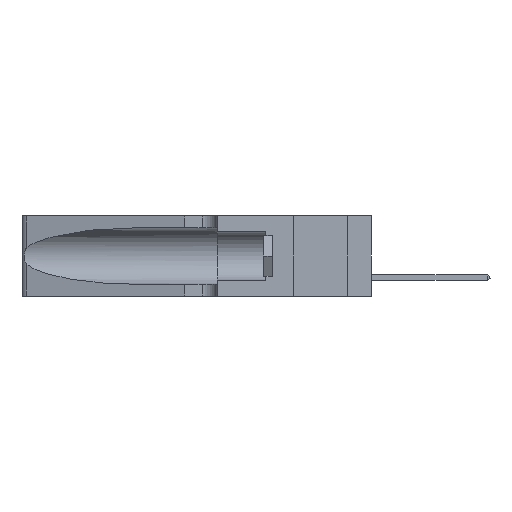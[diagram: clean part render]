
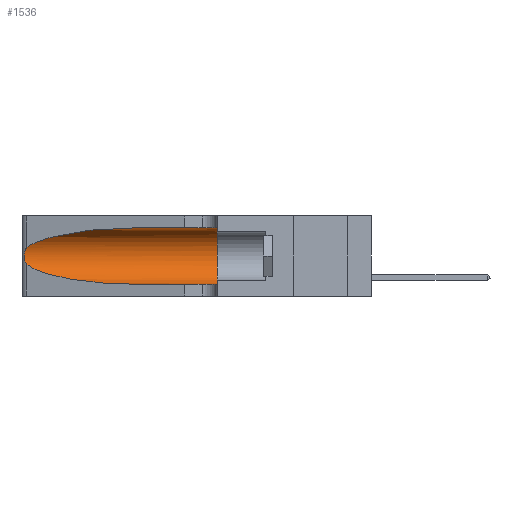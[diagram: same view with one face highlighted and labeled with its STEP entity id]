
A CAD part, left-side view. The second image highlights one B-rep face of the part: STEP entity #1536.
In plain terms, the highlighted cylindrical face has radius 3.308 mm (diameter 6.617 mm), a partial arc.
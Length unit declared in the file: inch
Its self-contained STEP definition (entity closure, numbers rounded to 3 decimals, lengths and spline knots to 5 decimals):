
#342 = CIRCLE ( 'NONE', #3537, 0.13025 ) ;
#1350 = EDGE_CURVE ( 'NONE', #8783, #22635, #342, .T. ) ;
#1366 = CARTESIAN_POINT ( 'NONE',  ( 0.1305, 0.35, 0.05475 ) ) ;
#1536 = ADVANCED_FACE ( 'NONE', ( #18230 ), #26900, .F. ) ;
#2215 = VERTEX_POINT ( 'NONE', #22317 ) ;
#2694 = CARTESIAN_POINT ( 'NONE',  ( 0.2373, 1.15595, 0.28018 ) ) ;
#3537 = AXIS2_PLACEMENT_3D ( 'NONE', #14195, #28420, #31105 ) ;
#4335 = EDGE_CURVE ( 'NONE', #12431, #22635, #7049, .T. ) ;
#4605 = CARTESIAN_POINT ( 'NONE',  ( 0.25487, 1.22718, 0.22369 ) ) ;
#4709 = VERTEX_POINT ( 'NONE', #4605 ) ;
#5006 = LINE ( 'NONE', #28798, #22879 ) ;
#6107 = EDGE_CURVE ( 'NONE', #7689, #8783, #5006, .T. ) ;
#6124 = CARTESIAN_POINT ( 'NONE',  ( 0.25789, 1.23486, 0.15765 ) ) ;
#6458 = CARTESIAN_POINT ( 'NONE',  ( 0.25854, 1.2359, 0.20912 ) ) ;
#6607 = EDGE_CURVE ( 'NONE', #7689, #4709, #11558, .T. ) ;
#7049 = LINE ( 'NONE', #31256, #7746 ) ;
#7689 = VERTEX_POINT ( 'NONE', #12386 ) ;
#7746 = VECTOR ( 'NONE', #16591, 39.37008 ) ;
#7882 = CARTESIAN_POINT ( 'NONE',  ( 0.18966, 0.96281, 0.05475 ) ) ;
#8782 = CARTESIAN_POINT ( 'NONE',  ( 0.25787, 1.23484, 0.2124 ) ) ;
#8783 = VERTEX_POINT ( 'NONE', #11712 ) ;
#10877 = CARTESIAN_POINT ( 'NONE',  ( 0.25555, 1.22993, 0.14849 ) ) ;
#11089 = CARTESIAN_POINT ( 'NONE',  ( 0.25639, 1.23184, 0.21858 ) ) ;
#11193 = CARTESIAN_POINT ( 'NONE',  ( 0.25639, 1.23186, 0.15144 ) ) ;
#11558 =( BOUNDED_CURVE ( )  B_SPLINE_CURVE ( 3, ( #31203, #24676, #2694, #17428 ),
 .UNSPECIFIED., .F., .F. ) 
 B_SPLINE_CURVE_WITH_KNOTS ( ( 4, 4 ),
 ( 1.5708, 2.84003 ),
 .UNSPECIFIED. ) 
 CURVE ( )  GEOMETRIC_REPRESENTATION_ITEM ( )  RATIONAL_B_SPLINE_CURVE ( ( 1., 0.87, 0.87, 1. ) ) 
 REPRESENTATION_ITEM ( '' )  );
#11678 = ORIENTED_EDGE ( 'NONE', *, *, #29140, .T. ) ;
#11712 = CARTESIAN_POINT ( 'NONE',  ( 0.1305, 0.35, 0.31525 ) ) ;
#11810 = ORIENTED_EDGE ( 'NONE', *, *, #21316, .T. ) ;
#12386 = CARTESIAN_POINT ( 'NONE',  ( 0.1305, 0.72297, 0.31525 ) ) ;
#12431 = VERTEX_POINT ( 'NONE', #30463 ) ;
#13354 = ORIENTED_EDGE ( 'NONE', *, *, #1350, .F. ) ;
#13398 = CARTESIAN_POINT ( 'NONE',  ( 0.25487, 1.22718, 0.14631 ) ) ;
#14097 = CARTESIAN_POINT ( 'NONE',  ( 0.1305, 1.61858, 0.185 ) ) ;
#14195 = CARTESIAN_POINT ( 'NONE',  ( 0.1305, 0.35, 0.185 ) ) ;
#14213 = DIRECTION ( 'NONE',  ( 0., -1., 0. ) ) ;
#14747 = CARTESIAN_POINT ( 'NONE',  ( 0.2373, 1.15595, 0.08982 ) ) ;
#15059 = AXIS2_PLACEMENT_3D ( 'NONE', #14097, #14213, #19146 ) ;
#16081 = CARTESIAN_POINT ( 'NONE',  ( 0.25856, 1.23593, 0.16098 ) ) ;
#16591 = DIRECTION ( 'NONE',  ( 0., -1., 0. ) ) ;
#16883 = DIRECTION ( 'NONE',  ( 0., -1., 0. ) ) ;
#17168 = B_SPLINE_CURVE_WITH_KNOTS ( 'NONE', 3,
 ( #23561, #28182, #11089, #8782, #6458, #23456, #30642, #20655, #25415, #16081, #6124, #11193, #10877, #13398 ),
 .UNSPECIFIED., .F., .F.,
 ( 4, 2, 2, 2, 2, 2, 4 ),
 ( 0., 0.00027, 0.00053, 0.00107, 0.0016, 0.00187, 0.00214 ),
 .UNSPECIFIED. ) ;
#17428 = CARTESIAN_POINT ( 'NONE',  ( 0.25487, 1.22718, 0.22369 ) ) ;
#18230 = FACE_OUTER_BOUND ( 'NONE', #22484, .T. ) ;
#19146 = DIRECTION ( 'NONE',  ( 0., 0., -1. ) ) ;
#20655 = CARTESIAN_POINT ( 'NONE',  ( 0.26075, 1.23896, 0.178 ) ) ;
#21316 = EDGE_CURVE ( 'NONE', #2215, #12431, #23280, .T. ) ;
#22025 = CARTESIAN_POINT ( 'NONE',  ( 0.25487, 1.22718, 0.14631 ) ) ;
#22317 = CARTESIAN_POINT ( 'NONE',  ( 0.25487, 1.22718, 0.14631 ) ) ;
#22484 = EDGE_LOOP ( 'NONE', ( #31211, #11678, #11810, #25449, #13354, #24732 ) ) ;
#22635 = VERTEX_POINT ( 'NONE', #1366 ) ;
#22879 = VECTOR ( 'NONE', #16883, 39.37008 ) ;
#23280 =( BOUNDED_CURVE ( )  B_SPLINE_CURVE ( 3, ( #22025, #14747, #7882, #24868 ),
 .UNSPECIFIED., .F., .F. ) 
 B_SPLINE_CURVE_WITH_KNOTS ( ( 4, 4 ),
 ( 3.44316, 4.71239 ),
 .UNSPECIFIED. ) 
 CURVE ( )  GEOMETRIC_REPRESENTATION_ITEM ( )  RATIONAL_B_SPLINE_CURVE ( ( 1., 0.87, 0.87, 1. ) ) 
 REPRESENTATION_ITEM ( '' )  );
#23456 = CARTESIAN_POINT ( 'NONE',  ( 0.26018, 1.23835, 0.19895 ) ) ;
#23561 = CARTESIAN_POINT ( 'NONE',  ( 0.25487, 1.22718, 0.22369 ) ) ;
#24676 = CARTESIAN_POINT ( 'NONE',  ( 0.18966, 0.96281, 0.31525 ) ) ;
#24732 = ORIENTED_EDGE ( 'NONE', *, *, #6107, .F. ) ;
#24868 = CARTESIAN_POINT ( 'NONE',  ( 0.1305, 0.72297, 0.05475 ) ) ;
#25415 = CARTESIAN_POINT ( 'NONE',  ( 0.26017, 1.23833, 0.17102 ) ) ;
#25449 = ORIENTED_EDGE ( 'NONE', *, *, #4335, .T. ) ;
#26900 = CYLINDRICAL_SURFACE ( 'NONE', #15059, 0.13025 ) ;
#28182 = CARTESIAN_POINT ( 'NONE',  ( 0.25555, 1.22994, 0.2215 ) ) ;
#28420 = DIRECTION ( 'NONE',  ( 0., 1., 0. ) ) ;
#28798 = CARTESIAN_POINT ( 'NONE',  ( 0.1305, 1.61858, 0.31525 ) ) ;
#29140 = EDGE_CURVE ( 'NONE', #4709, #2215, #17168, .T. ) ;
#30463 = CARTESIAN_POINT ( 'NONE',  ( 0.1305, 0.72297, 0.05475 ) ) ;
#30642 = CARTESIAN_POINT ( 'NONE',  ( 0.26075, 1.23896, 0.19203 ) ) ;
#31105 = DIRECTION ( 'NONE',  ( 0., 0., 1. ) ) ;
#31203 = CARTESIAN_POINT ( 'NONE',  ( 0.1305, 0.72297, 0.31525 ) ) ;
#31211 = ORIENTED_EDGE ( 'NONE', *, *, #6607, .T. ) ;
#31256 = CARTESIAN_POINT ( 'NONE',  ( 0.1305, 1.61858, 0.05475 ) ) ;
